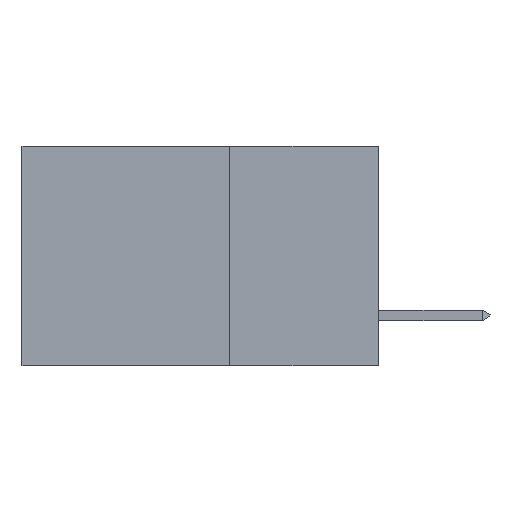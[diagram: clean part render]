
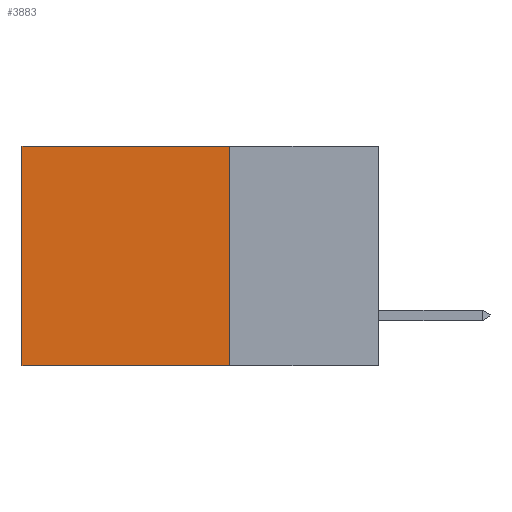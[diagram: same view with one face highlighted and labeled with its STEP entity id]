
A CAD part, left-side view. The second image highlights one B-rep face of the part: STEP entity #3883.
In plain terms, the highlighted planar face has unit normal (-1, 0, 0).
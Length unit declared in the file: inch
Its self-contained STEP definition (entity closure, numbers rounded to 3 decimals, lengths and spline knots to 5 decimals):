
#335 = EDGE_CURVE ( 'NONE', #6157, #3188, #6231, .T. ) ;
#484 = PLANE ( 'NONE',  #3045 ) ;
#570 = VECTOR ( 'NONE', #9058, 39.37008 ) ;
#1231 = VECTOR ( 'NONE', #5033, 39.37008 ) ;
#1250 = DIRECTION ( 'NONE',  ( 0., 1., 0. ) ) ;
#1830 = CARTESIAN_POINT ( 'NONE',  ( 0.298, 0.25, -0.37 ) ) ;
#1851 = CARTESIAN_POINT ( 'NONE',  ( 0.298, 0.25, -0.37 ) ) ;
#2102 = CARTESIAN_POINT ( 'NONE',  ( 0.298, 0.25, 0. ) ) ;
#2744 = CARTESIAN_POINT ( 'NONE',  ( 0.298, 0.25, 0. ) ) ;
#2850 = EDGE_LOOP ( 'NONE', ( #9168, #9592, #6559, #6072 ) ) ;
#2857 = EDGE_CURVE ( 'NONE', #3705, #3188, #11076, .T. ) ;
#3045 = AXIS2_PLACEMENT_3D ( 'NONE', #6845, #11473, #6092 ) ;
#3188 = VERTEX_POINT ( 'NONE', #9560 ) ;
#3705 = VERTEX_POINT ( 'NONE', #4608 ) ;
#3883 = ADVANCED_FACE ( 'NONE', ( #7713 ), #484, .F. ) ;
#4151 = EDGE_CURVE ( 'NONE', #7565, #3705, #7429, .T. ) ;
#4608 = CARTESIAN_POINT ( 'NONE',  ( 0.298, 0.6, 0. ) ) ;
#5033 = DIRECTION ( 'NONE',  ( 0., 0., -1. ) ) ;
#5301 = LINE ( 'NONE', #2744, #9281 ) ;
#6072 = ORIENTED_EDGE ( 'NONE', *, *, #4151, .T. ) ;
#6092 = DIRECTION ( 'NONE',  ( 0., 0., -1. ) ) ;
#6157 = VERTEX_POINT ( 'NONE', #1830 ) ;
#6231 = LINE ( 'NONE', #1851, #570 ) ;
#6559 = ORIENTED_EDGE ( 'NONE', *, *, #10081, .F. ) ;
#6826 = VECTOR ( 'NONE', #1250, 39.37008 ) ;
#6845 = CARTESIAN_POINT ( 'NONE',  ( 0.298, 0.25, 0. ) ) ;
#7429 = LINE ( 'NONE', #2102, #6826 ) ;
#7565 = VERTEX_POINT ( 'NONE', #10918 ) ;
#7713 = FACE_OUTER_BOUND ( 'NONE', #2850, .T. ) ;
#8661 = CARTESIAN_POINT ( 'NONE',  ( 0.298, 0.6, 0. ) ) ;
#9058 = DIRECTION ( 'NONE',  ( 0., 1., 0. ) ) ;
#9168 = ORIENTED_EDGE ( 'NONE', *, *, #2857, .T. ) ;
#9281 = VECTOR ( 'NONE', #9948, 39.37008 ) ;
#9560 = CARTESIAN_POINT ( 'NONE',  ( 0.298, 0.6, -0.37 ) ) ;
#9592 = ORIENTED_EDGE ( 'NONE', *, *, #335, .F. ) ;
#9948 = DIRECTION ( 'NONE',  ( 0., 0., -1. ) ) ;
#10081 = EDGE_CURVE ( 'NONE', #7565, #6157, #5301, .T. ) ;
#10918 = CARTESIAN_POINT ( 'NONE',  ( 0.298, 0.25, 0. ) ) ;
#11076 = LINE ( 'NONE', #8661, #1231 ) ;
#11473 = DIRECTION ( 'NONE',  ( 1., 0., 0. ) ) ;
